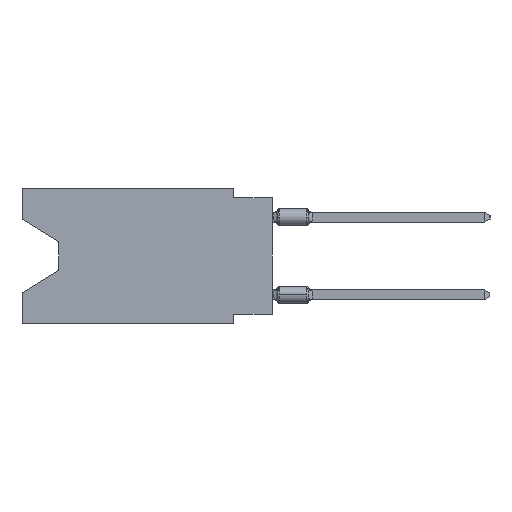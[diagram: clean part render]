
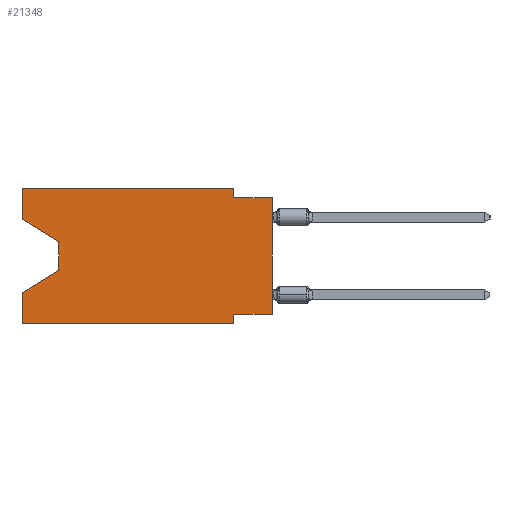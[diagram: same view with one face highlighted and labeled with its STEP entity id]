
A CAD part, left-side view. The second image highlights one B-rep face of the part: STEP entity #21348.
In plain terms, the highlighted planar face has unit normal (-1, 0, 0).
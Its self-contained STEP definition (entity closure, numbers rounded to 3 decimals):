
#639 = CARTESIAN_POINT ( 'NONE',  ( 0., 0., -0.635 ) ) ;
#811 = CARTESIAN_POINT ( 'NONE',  ( 0., 0., -0.635 ) ) ;
#999 = DIRECTION ( 'NONE',  ( 0., -1., 0. ) ) ;
#1094 = EDGE_CURVE ( 'NONE', #15015, #23985, #27471, .T. ) ;
#1484 = EDGE_LOOP ( 'NONE', ( #20007, #31907, #18288, #3115, #14666, #19951, #21310, #20126, #8741, #7205, #25361, #12688 ) ) ;
#1899 = CARTESIAN_POINT ( 'NONE',  ( 0., 16.383, -8.89 ) ) ;
#2061 = DIRECTION ( 'NONE',  ( 1., 0., 0. ) ) ;
#3115 = ORIENTED_EDGE ( 'NONE', *, *, #31808, .F. ) ;
#3119 = DIRECTION ( 'NONE',  ( 0., 0., -1. ) ) ;
#3201 = VERTEX_POINT ( 'NONE', #11604 ) ;
#3484 = CARTESIAN_POINT ( 'NONE',  ( 0., 16.383, -2.038 ) ) ;
#3823 = VERTEX_POINT ( 'NONE', #15899 ) ;
#3842 = LINE ( 'NONE', #3484, #11731 ) ;
#3863 = DIRECTION ( 'NONE',  ( 0., 1., 0. ) ) ;
#4425 = EDGE_CURVE ( 'NONE', #22833, #35302, #33140, .T. ) ;
#4496 = DIRECTION ( 'NONE',  ( 0., 0., -1. ) ) ;
#4594 = DIRECTION ( 'NONE',  ( 0., 0., -1. ) ) ;
#5089 = LINE ( 'NONE', #24785, #24725 ) ;
#5148 = EDGE_CURVE ( 'NONE', #6648, #22833, #3842, .T. ) ;
#5806 = CARTESIAN_POINT ( 'NONE',  ( 0., 16.383, 0. ) ) ;
#6648 = VERTEX_POINT ( 'NONE', #8961 ) ;
#6937 = LINE ( 'NONE', #34248, #35415 ) ;
#7205 = ORIENTED_EDGE ( 'NONE', *, *, #10853, .F. ) ;
#8230 = CARTESIAN_POINT ( 'NONE',  ( 0., 2.54, 0. ) ) ;
#8741 = ORIENTED_EDGE ( 'NONE', *, *, #19882, .F. ) ;
#8961 = CARTESIAN_POINT ( 'NONE',  ( 0., 16.383, -2.038 ) ) ;
#9059 = LINE ( 'NONE', #5806, #9815 ) ;
#9815 = VECTOR ( 'NONE', #17197, 1000. ) ;
#10586 = LINE ( 'NONE', #8230, #29327 ) ;
#10853 = EDGE_CURVE ( 'NONE', #26790, #15755, #10586, .T. ) ;
#10895 = VECTOR ( 'NONE', #23036, 1000. ) ;
#11433 = VERTEX_POINT ( 'NONE', #23181 ) ;
#11604 = CARTESIAN_POINT ( 'NONE',  ( 0., 16.383, 0. ) ) ;
#11665 = EDGE_CURVE ( 'NONE', #28868, #11433, #5089, .T. ) ;
#11731 = VECTOR ( 'NONE', #28794, 1000. ) ;
#12004 = LINE ( 'NONE', #23571, #10895 ) ;
#12688 = ORIENTED_EDGE ( 'NONE', *, *, #33234, .F. ) ;
#13801 = EDGE_CURVE ( 'NONE', #35302, #16380, #17230, .T. ) ;
#13980 = DIRECTION ( 'NONE',  ( 0., 0.855, -0.519 ) ) ;
#14666 = ORIENTED_EDGE ( 'NONE', *, *, #11665, .T. ) ;
#15015 = VERTEX_POINT ( 'NONE', #24411 ) ;
#15350 = CARTESIAN_POINT ( 'NONE',  ( 0., 2.54, -8.89 ) ) ;
#15755 = VERTEX_POINT ( 'NONE', #22451 ) ;
#15799 = CARTESIAN_POINT ( 'NONE',  ( 0., 16.383, 0. ) ) ;
#15899 = CARTESIAN_POINT ( 'NONE',  ( 0., 2.54, -8.255 ) ) ;
#16380 = VERTEX_POINT ( 'NONE', #31628 ) ;
#16840 = CARTESIAN_POINT ( 'NONE',  ( 0., 16.383, 0. ) ) ;
#17197 = DIRECTION ( 'NONE',  ( 0., 0., 1. ) ) ;
#17230 = LINE ( 'NONE', #27898, #30301 ) ;
#18044 = EDGE_CURVE ( 'NONE', #3823, #11433, #18242, .T. ) ;
#18242 = LINE ( 'NONE', #15350, #18743 ) ;
#18288 = ORIENTED_EDGE ( 'NONE', *, *, #13801, .T. ) ;
#18302 = CARTESIAN_POINT ( 'NONE',  ( 0., 13.97, -3.505 ) ) ;
#18331 = EDGE_CURVE ( 'NONE', #15015, #3823, #6937, .T. ) ;
#18743 = VECTOR ( 'NONE', #4496, 1000. ) ;
#18989 = VECTOR ( 'NONE', #25513, 1000. ) ;
#19212 = VECTOR ( 'NONE', #999, 1000. ) ;
#19882 = EDGE_CURVE ( 'NONE', #15755, #23985, #33389, .T. ) ;
#19951 = ORIENTED_EDGE ( 'NONE', *, *, #18044, .F. ) ;
#20007 = ORIENTED_EDGE ( 'NONE', *, *, #5148, .T. ) ;
#20126 = ORIENTED_EDGE ( 'NONE', *, *, #1094, .T. ) ;
#20776 = VECTOR ( 'NONE', #30363, 1000. ) ;
#21310 = ORIENTED_EDGE ( 'NONE', *, *, #18331, .F. ) ;
#21348 = ADVANCED_FACE ( 'NONE', ( #29009 ), #26290, .F. ) ;
#22182 = AXIS2_PLACEMENT_3D ( 'NONE', #15799, #2061, #4594 ) ;
#22451 = CARTESIAN_POINT ( 'NONE',  ( 0., 2.54, -0.635 ) ) ;
#22833 = VERTEX_POINT ( 'NONE', #18302 ) ;
#23036 = DIRECTION ( 'NONE',  ( 0., -1., 0. ) ) ;
#23181 = CARTESIAN_POINT ( 'NONE',  ( 0., 2.54, -8.89 ) ) ;
#23571 = CARTESIAN_POINT ( 'NONE',  ( 0., 16.383, 0. ) ) ;
#23985 = VERTEX_POINT ( 'NONE', #811 ) ;
#24410 = VECTOR ( 'NONE', #3119, 1000. ) ;
#24411 = CARTESIAN_POINT ( 'NONE',  ( 0., 0., -8.255 ) ) ;
#24725 = VECTOR ( 'NONE', #33639, 1000. ) ;
#24785 = CARTESIAN_POINT ( 'NONE',  ( 0., 16.383, -8.89 ) ) ;
#24866 = DIRECTION ( 'NONE',  ( 0., 0., -1. ) ) ;
#24998 = CARTESIAN_POINT ( 'NONE',  ( 0., 13.97, -3.505 ) ) ;
#25361 = ORIENTED_EDGE ( 'NONE', *, *, #31657, .F. ) ;
#25513 = DIRECTION ( 'NONE',  ( 0., 0., 1. ) ) ;
#26290 = PLANE ( 'NONE',  #22182 ) ;
#26790 = VERTEX_POINT ( 'NONE', #33574 ) ;
#27471 = LINE ( 'NONE', #35259, #20776 ) ;
#27898 = CARTESIAN_POINT ( 'NONE',  ( 0., 13.97, -5.385 ) ) ;
#28794 = DIRECTION ( 'NONE',  ( 0., -0.855, -0.519 ) ) ;
#28868 = VERTEX_POINT ( 'NONE', #1899 ) ;
#29009 = FACE_OUTER_BOUND ( 'NONE', #1484, .T. ) ;
#29327 = VECTOR ( 'NONE', #24866, 1000. ) ;
#30237 = LINE ( 'NONE', #16840, #18989 ) ;
#30301 = VECTOR ( 'NONE', #13980, 1000. ) ;
#30363 = DIRECTION ( 'NONE',  ( 0., 0., 1. ) ) ;
#31628 = CARTESIAN_POINT ( 'NONE',  ( 0., 16.383, -6.852 ) ) ;
#31657 = EDGE_CURVE ( 'NONE', #3201, #26790, #12004, .T. ) ;
#31808 = EDGE_CURVE ( 'NONE', #28868, #16380, #30237, .T. ) ;
#31907 = ORIENTED_EDGE ( 'NONE', *, *, #4425, .T. ) ;
#33040 = CARTESIAN_POINT ( 'NONE',  ( 0., 13.97, -5.385 ) ) ;
#33140 = LINE ( 'NONE', #24998, #24410 ) ;
#33234 = EDGE_CURVE ( 'NONE', #6648, #3201, #9059, .T. ) ;
#33389 = LINE ( 'NONE', #639, #19212 ) ;
#33574 = CARTESIAN_POINT ( 'NONE',  ( 0., 2.54, 0. ) ) ;
#33639 = DIRECTION ( 'NONE',  ( 0., -1., 0. ) ) ;
#34248 = CARTESIAN_POINT ( 'NONE',  ( 0., 0., -8.255 ) ) ;
#35259 = CARTESIAN_POINT ( 'NONE',  ( 0., 0., 0. ) ) ;
#35302 = VERTEX_POINT ( 'NONE', #33040 ) ;
#35415 = VECTOR ( 'NONE', #3863, 1000. ) ;
